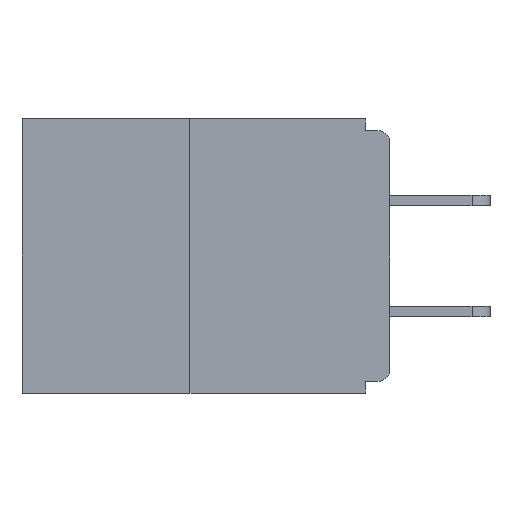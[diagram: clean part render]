
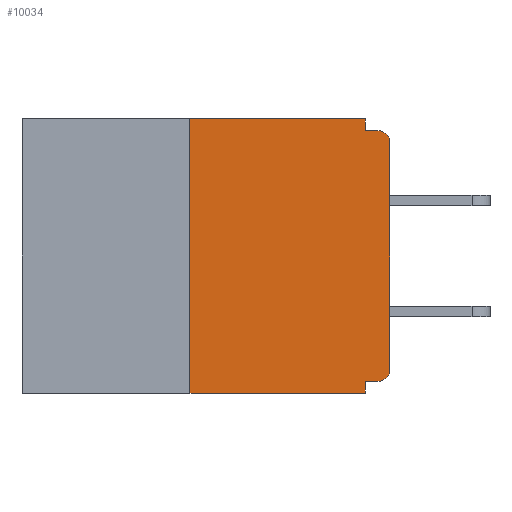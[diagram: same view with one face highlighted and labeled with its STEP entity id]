
A CAD part, left-side view. The second image highlights one B-rep face of the part: STEP entity #10034.
In plain terms, the highlighted planar face has unit normal (-1, 0, 0).
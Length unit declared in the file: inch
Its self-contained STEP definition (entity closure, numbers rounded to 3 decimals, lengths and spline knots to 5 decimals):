
#29 = VERTEX_POINT ( 'NONE', #20352 ) ;
#476 = CARTESIAN_POINT ( 'NONE',  ( 0., 0., -0.328 ) ) ;
#543 = CARTESIAN_POINT ( 'NONE',  ( 0., 0.031, -0.343 ) ) ;
#631 = EDGE_CURVE ( 'NONE', #13064, #17766, #5496, .T. ) ;
#640 = VERTEX_POINT ( 'NONE', #16063 ) ;
#700 = VECTOR ( 'NONE', #4219, 39.37008 ) ;
#1163 = DIRECTION ( 'NONE',  ( -1., 0., 0. ) ) ;
#1275 = ORIENTED_EDGE ( 'NONE', *, *, #631, .T. ) ;
#1678 = CARTESIAN_POINT ( 'NONE',  ( 0., 0.031, 0. ) ) ;
#1847 = LINE ( 'NONE', #476, #7025 ) ;
#1870 = VECTOR ( 'NONE', #19575, 39.37008 ) ;
#1890 = VERTEX_POINT ( 'NONE', #19723 ) ;
#2283 = ORIENTED_EDGE ( 'NONE', *, *, #16311, .F. ) ;
#2382 = CARTESIAN_POINT ( 'NONE',  ( 0., 0.25, 0. ) ) ;
#2414 = CARTESIAN_POINT ( 'NONE',  ( 0., 0.031, 0. ) ) ;
#3094 = LINE ( 'NONE', #5981, #13711 ) ;
#3414 = EDGE_CURVE ( 'NONE', #3435, #16324, #15188, .T. ) ;
#3435 = VERTEX_POINT ( 'NONE', #2382 ) ;
#3543 = VECTOR ( 'NONE', #12673, 39.37008 ) ;
#3722 = EDGE_CURVE ( 'NONE', #17766, #29, #12569, .T. ) ;
#3739 = AXIS2_PLACEMENT_3D ( 'NONE', #7871, #1163, #20969 ) ;
#3794 = CARTESIAN_POINT ( 'NONE',  ( 0., 0.25, -0.343 ) ) ;
#4219 = DIRECTION ( 'NONE',  ( 0., -1., 0. ) ) ;
#4490 = EDGE_CURVE ( 'NONE', #10851, #16282, #16223, .T. ) ;
#5317 = DIRECTION ( 'NONE',  ( 0., 1., 0. ) ) ;
#5496 = CIRCLE ( 'NONE', #10411, 0.015 ) ;
#5649 = ORIENTED_EDGE ( 'NONE', *, *, #16438, .T. ) ;
#5981 = CARTESIAN_POINT ( 'NONE',  ( 0., 0., -0.015 ) ) ;
#6409 = CARTESIAN_POINT ( 'NONE',  ( 0., 0.25, 0. ) ) ;
#6493 = CARTESIAN_POINT ( 'NONE',  ( 0., 0.031, -0.328 ) ) ;
#6996 = LINE ( 'NONE', #13423, #19763 ) ;
#7025 = VECTOR ( 'NONE', #5317, 39.37008 ) ;
#7871 = CARTESIAN_POINT ( 'NONE',  ( 0., 0.015, -0.03 ) ) ;
#7935 = CARTESIAN_POINT ( 'NONE',  ( 0., 0.015, -0.313 ) ) ;
#8317 = CARTESIAN_POINT ( 'NONE',  ( 0., 0., -0.313 ) ) ;
#8331 = DIRECTION ( 'NONE',  ( 0., 0., -1. ) ) ;
#8920 = CARTESIAN_POINT ( 'NONE',  ( 0., 0.46, -0.343 ) ) ;
#9024 = CARTESIAN_POINT ( 'NONE',  ( 0., 0.46, 0. ) ) ;
#9273 = DIRECTION ( 'NONE',  ( 0., -1., 0. ) ) ;
#9451 = ORIENTED_EDGE ( 'NONE', *, *, #19580, .F. ) ;
#9468 = EDGE_CURVE ( 'NONE', #10291, #16282, #6996, .T. ) ;
#9821 = DIRECTION ( 'NONE',  ( 0., 0., -1. ) ) ;
#10034 = ADVANCED_FACE ( 'NONE', ( #11846 ), #10861, .F. ) ;
#10291 = VERTEX_POINT ( 'NONE', #6493 ) ;
#10366 = LINE ( 'NONE', #6409, #1870 ) ;
#10411 = AXIS2_PLACEMENT_3D ( 'NONE', #7935, #16130, #14525 ) ;
#10851 = VERTEX_POINT ( 'NONE', #3794 ) ;
#10861 = PLANE ( 'NONE',  #18448 ) ;
#11196 = ORIENTED_EDGE ( 'NONE', *, *, #9468, .F. ) ;
#11846 = FACE_OUTER_BOUND ( 'NONE', #20460, .T. ) ;
#12347 = CARTESIAN_POINT ( 'NONE',  ( 0., 0.46, 0. ) ) ;
#12569 = LINE ( 'NONE', #20972, #3543 ) ;
#12673 = DIRECTION ( 'NONE',  ( 0., 0., 1. ) ) ;
#12691 = ORIENTED_EDGE ( 'NONE', *, *, #3722, .T. ) ;
#12706 = CIRCLE ( 'NONE', #3739, 0.015 ) ;
#13064 = VERTEX_POINT ( 'NONE', #15030 ) ;
#13423 = CARTESIAN_POINT ( 'NONE',  ( 0., 0.031, -0.343 ) ) ;
#13711 = VECTOR ( 'NONE', #9273, 39.37008 ) ;
#13965 = DIRECTION ( 'NONE',  ( 1., 0., 0. ) ) ;
#14164 = VECTOR ( 'NONE', #15690, 39.37008 ) ;
#14243 = EDGE_CURVE ( 'NONE', #16324, #1890, #18021, .T. ) ;
#14525 = DIRECTION ( 'NONE',  ( 0., 0., -1. ) ) ;
#15030 = CARTESIAN_POINT ( 'NONE',  ( 0., 0.015, -0.328 ) ) ;
#15188 = LINE ( 'NONE', #9024, #14164 ) ;
#15690 = DIRECTION ( 'NONE',  ( 0., -1., 0. ) ) ;
#16063 = CARTESIAN_POINT ( 'NONE',  ( 0., 0.015, -0.015 ) ) ;
#16130 = DIRECTION ( 'NONE',  ( -1., 0., 0. ) ) ;
#16143 = ORIENTED_EDGE ( 'NONE', *, *, #4490, .T. ) ;
#16223 = LINE ( 'NONE', #8920, #700 ) ;
#16282 = VERTEX_POINT ( 'NONE', #543 ) ;
#16311 = EDGE_CURVE ( 'NONE', #13064, #10291, #1847, .T. ) ;
#16324 = VERTEX_POINT ( 'NONE', #2414 ) ;
#16438 = EDGE_CURVE ( 'NONE', #29, #640, #12706, .T. ) ;
#16635 = ORIENTED_EDGE ( 'NONE', *, *, #14243, .F. ) ;
#17070 = EDGE_CURVE ( 'NONE', #1890, #640, #3094, .T. ) ;
#17766 = VERTEX_POINT ( 'NONE', #8317 ) ;
#18021 = LINE ( 'NONE', #1678, #21457 ) ;
#18448 = AXIS2_PLACEMENT_3D ( 'NONE', #12347, #13965, #20648 ) ;
#19480 = ORIENTED_EDGE ( 'NONE', *, *, #17070, .F. ) ;
#19575 = DIRECTION ( 'NONE',  ( 0., 0., 1. ) ) ;
#19580 = EDGE_CURVE ( 'NONE', #10851, #3435, #10366, .T. ) ;
#19723 = CARTESIAN_POINT ( 'NONE',  ( 0., 0.031, -0.015 ) ) ;
#19763 = VECTOR ( 'NONE', #8331, 39.37008 ) ;
#20323 = ORIENTED_EDGE ( 'NONE', *, *, #3414, .F. ) ;
#20352 = CARTESIAN_POINT ( 'NONE',  ( 0., 0., -0.03 ) ) ;
#20460 = EDGE_LOOP ( 'NONE', ( #20323, #9451, #16143, #11196, #2283, #1275, #12691, #5649, #19480, #16635 ) ) ;
#20648 = DIRECTION ( 'NONE',  ( 0., 0., -1. ) ) ;
#20969 = DIRECTION ( 'NONE',  ( 0., 0., -1. ) ) ;
#20972 = CARTESIAN_POINT ( 'NONE',  ( 0., 0., 0. ) ) ;
#21457 = VECTOR ( 'NONE', #9821, 39.37008 ) ;
